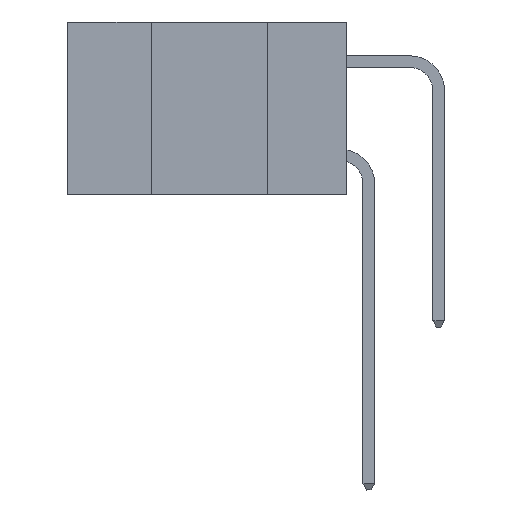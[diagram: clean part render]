
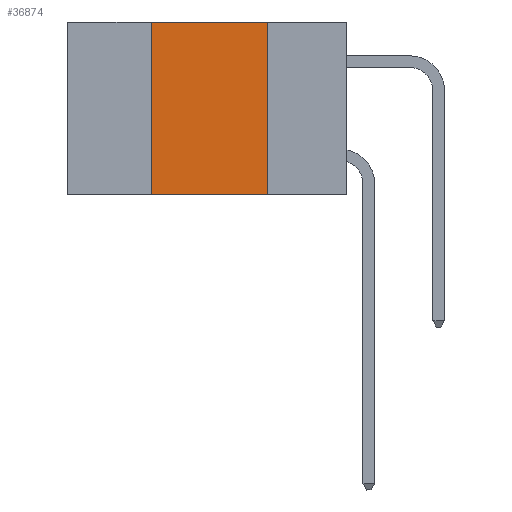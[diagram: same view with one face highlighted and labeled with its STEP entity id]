
A CAD part, left-side view. The second image highlights one B-rep face of the part: STEP entity #36874.
In plain terms, the highlighted planar face has unit normal (-1, 0, 0).
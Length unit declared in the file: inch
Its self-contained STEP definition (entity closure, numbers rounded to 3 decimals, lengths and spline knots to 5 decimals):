
#60 = DIRECTION ( 'NONE',  ( 0., -1., 0. ) ) ;
#531 = VECTOR ( 'NONE', #26872, 39.37008 ) ;
#1688 = EDGE_LOOP ( 'NONE', ( #26926, #30266, #24439, #15096 ) ) ;
#2847 = CARTESIAN_POINT ( 'NONE',  ( 0., 0.17, -0.37 ) ) ;
#3565 = VERTEX_POINT ( 'NONE', #12509 ) ;
#5898 = LINE ( 'NONE', #38922, #20946 ) ;
#7010 = CARTESIAN_POINT ( 'NONE',  ( 0., 0.17, 0. ) ) ;
#9094 = CARTESIAN_POINT ( 'NONE',  ( 0., 0.6, 0. ) ) ;
#9371 = PLANE ( 'NONE',  #17092 ) ;
#10022 = CARTESIAN_POINT ( 'NONE',  ( 0., 0.42, -0.37 ) ) ;
#11807 = DIRECTION ( 'NONE',  ( 0., 0., 1. ) ) ;
#12509 = CARTESIAN_POINT ( 'NONE',  ( 0., 0.42, 0. ) ) ;
#14420 = LINE ( 'NONE', #33781, #21179 ) ;
#15096 = ORIENTED_EDGE ( 'NONE', *, *, #31814, .T. ) ;
#16209 = VERTEX_POINT ( 'NONE', #7010 ) ;
#17092 = AXIS2_PLACEMENT_3D ( 'NONE', #9094, #22504, #22938 ) ;
#17972 = LINE ( 'NONE', #33095, #33593 ) ;
#18250 = LINE ( 'NONE', #39430, #531 ) ;
#20946 = VECTOR ( 'NONE', #11807, 39.37008 ) ;
#21179 = VECTOR ( 'NONE', #60, 39.37008 ) ;
#22504 = DIRECTION ( 'NONE',  ( 1., 0., 0. ) ) ;
#22938 = DIRECTION ( 'NONE',  ( 0., 0., -1. ) ) ;
#24439 = ORIENTED_EDGE ( 'NONE', *, *, #42215, .F. ) ;
#26872 = DIRECTION ( 'NONE',  ( 0., -1., 0. ) ) ;
#26926 = ORIENTED_EDGE ( 'NONE', *, *, #33573, .F. ) ;
#28900 = VERTEX_POINT ( 'NONE', #10022 ) ;
#30266 = ORIENTED_EDGE ( 'NONE', *, *, #36407, .F. ) ;
#31814 = EDGE_CURVE ( 'NONE', #28900, #36882, #14420, .T. ) ;
#33095 = CARTESIAN_POINT ( 'NONE',  ( 0., 0.17, 0. ) ) ;
#33573 = EDGE_CURVE ( 'NONE', #16209, #36882, #17972, .T. ) ;
#33593 = VECTOR ( 'NONE', #36473, 39.37008 ) ;
#33781 = CARTESIAN_POINT ( 'NONE',  ( 0., 0.6, -0.37 ) ) ;
#35410 = FACE_OUTER_BOUND ( 'NONE', #1688, .T. ) ;
#36407 = EDGE_CURVE ( 'NONE', #3565, #16209, #18250, .T. ) ;
#36473 = DIRECTION ( 'NONE',  ( 0., 0., -1. ) ) ;
#36874 = ADVANCED_FACE ( 'NONE', ( #35410 ), #9371, .F. ) ;
#36882 = VERTEX_POINT ( 'NONE', #2847 ) ;
#38922 = CARTESIAN_POINT ( 'NONE',  ( 0., 0.42, 0. ) ) ;
#39430 = CARTESIAN_POINT ( 'NONE',  ( 0., 0.6, 0. ) ) ;
#42215 = EDGE_CURVE ( 'NONE', #28900, #3565, #5898, .T. ) ;
